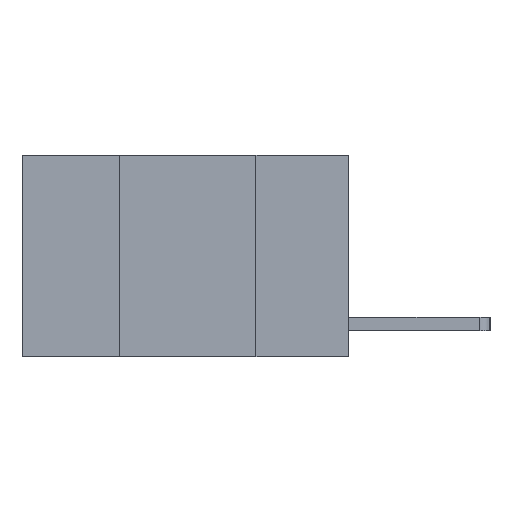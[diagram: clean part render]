
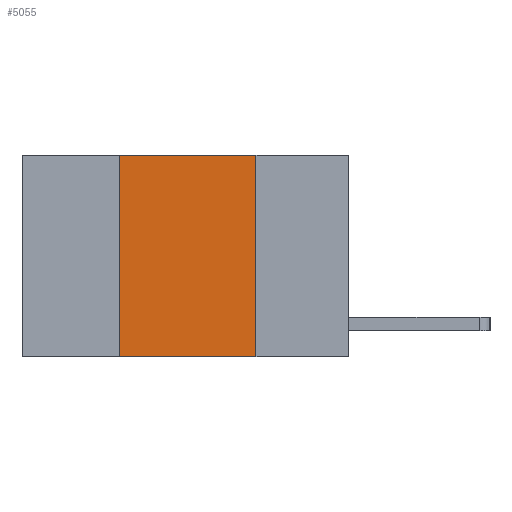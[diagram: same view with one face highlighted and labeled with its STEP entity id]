
A CAD part, left-side view. The second image highlights one B-rep face of the part: STEP entity #5055.
In plain terms, the highlighted planar face has unit normal (-1, 0, 0).
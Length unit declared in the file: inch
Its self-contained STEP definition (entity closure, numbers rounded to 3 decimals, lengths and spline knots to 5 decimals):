
#46 = VECTOR ( 'NONE', #3761, 39.37008 ) ;
#196 = LINE ( 'NONE', #5599, #4236 ) ;
#474 = EDGE_CURVE ( 'NONE', #5561, #7385, #847, .T. ) ;
#847 = LINE ( 'NONE', #7774, #2446 ) ;
#888 = CARTESIAN_POINT ( 'NONE',  ( 0., 0.6, 0. ) ) ;
#1188 = LINE ( 'NONE', #8334, #7531 ) ;
#1449 = VERTEX_POINT ( 'NONE', #3191 ) ;
#1664 = VERTEX_POINT ( 'NONE', #5839 ) ;
#1960 = ORIENTED_EDGE ( 'NONE', *, *, #474, .T. ) ;
#1974 = CARTESIAN_POINT ( 'NONE',  ( 0., 0.17, -0.37 ) ) ;
#2409 = DIRECTION ( 'NONE',  ( 0., 0., -1. ) ) ;
#2446 = VECTOR ( 'NONE', #7709, 39.37008 ) ;
#2466 = PLANE ( 'NONE',  #6036 ) ;
#2496 = FACE_OUTER_BOUND ( 'NONE', #6504, .T. ) ;
#3191 = CARTESIAN_POINT ( 'NONE',  ( 0., 0.42, 0. ) ) ;
#3643 = EDGE_CURVE ( 'NONE', #5561, #1449, #1188, .T. ) ;
#3761 = DIRECTION ( 'NONE',  ( 0., -1., 0. ) ) ;
#4236 = VECTOR ( 'NONE', #2409, 39.37008 ) ;
#4358 = DIRECTION ( 'NONE',  ( 0., 0., 1. ) ) ;
#4433 = ORIENTED_EDGE ( 'NONE', *, *, #8357, .F. ) ;
#4654 = ORIENTED_EDGE ( 'NONE', *, *, #3643, .F. ) ;
#4892 = DIRECTION ( 'NONE',  ( 0., 0., -1. ) ) ;
#5055 = ADVANCED_FACE ( 'NONE', ( #2496 ), #2466, .F. ) ;
#5554 = ORIENTED_EDGE ( 'NONE', *, *, #9450, .F. ) ;
#5561 = VERTEX_POINT ( 'NONE', #7038 ) ;
#5599 = CARTESIAN_POINT ( 'NONE',  ( 0., 0.17, 0. ) ) ;
#5839 = CARTESIAN_POINT ( 'NONE',  ( 0., 0.17, 0. ) ) ;
#6036 = AXIS2_PLACEMENT_3D ( 'NONE', #888, #9651, #4892 ) ;
#6504 = EDGE_LOOP ( 'NONE', ( #4433, #5554, #4654, #1960 ) ) ;
#7038 = CARTESIAN_POINT ( 'NONE',  ( 0., 0.42, -0.37 ) ) ;
#7385 = VERTEX_POINT ( 'NONE', #1974 ) ;
#7531 = VECTOR ( 'NONE', #4358, 39.37008 ) ;
#7709 = DIRECTION ( 'NONE',  ( 0., -1., 0. ) ) ;
#7774 = CARTESIAN_POINT ( 'NONE',  ( 0., 0.6, -0.37 ) ) ;
#8334 = CARTESIAN_POINT ( 'NONE',  ( 0., 0.42, 0. ) ) ;
#8357 = EDGE_CURVE ( 'NONE', #1664, #7385, #196, .T. ) ;
#8590 = LINE ( 'NONE', #10117, #46 ) ;
#9450 = EDGE_CURVE ( 'NONE', #1449, #1664, #8590, .T. ) ;
#9651 = DIRECTION ( 'NONE',  ( 1., 0., 0. ) ) ;
#10117 = CARTESIAN_POINT ( 'NONE',  ( 0., 0.6, 0. ) ) ;
